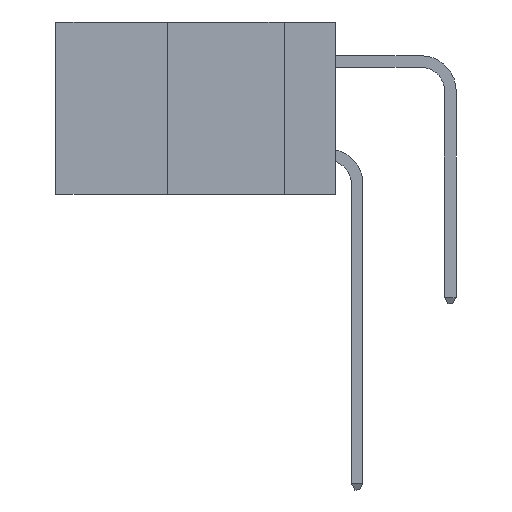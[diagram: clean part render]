
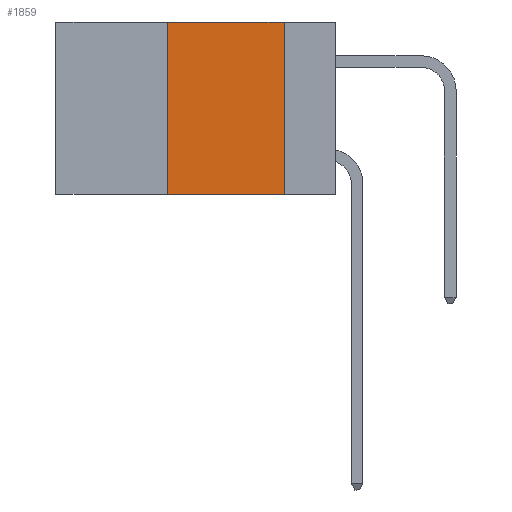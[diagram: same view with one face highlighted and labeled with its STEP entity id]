
A CAD part, left-side view. The second image highlights one B-rep face of the part: STEP entity #1859.
In plain terms, the highlighted planar face has unit normal (-1, 0, 0).
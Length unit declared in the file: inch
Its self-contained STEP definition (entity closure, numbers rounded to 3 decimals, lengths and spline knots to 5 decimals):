
#410 = VERTEX_POINT ( 'NONE', #22823 ) ;
#966 = EDGE_CURVE ( 'NONE', #22401, #4072, #22796, .T. ) ;
#1194 = CARTESIAN_POINT ( 'NONE',  ( 0., 0.11, 0. ) ) ;
#1469 = PLANE ( 'NONE',  #1845 ) ;
#1845 = AXIS2_PLACEMENT_3D ( 'NONE', #17821, #3337, #16053 ) ;
#1859 = ADVANCED_FACE ( 'NONE', ( #3425 ), #1469, .F. ) ;
#3337 = DIRECTION ( 'NONE',  ( 1., 0., 0. ) ) ;
#3425 = FACE_OUTER_BOUND ( 'NONE', #22972, .T. ) ;
#4072 = VERTEX_POINT ( 'NONE', #20283 ) ;
#4544 = CARTESIAN_POINT ( 'NONE',  ( 0., 0.11, 0. ) ) ;
#4611 = LINE ( 'NONE', #4544, #5171 ) ;
#5171 = VECTOR ( 'NONE', #17286, 39.37008 ) ;
#5440 = DIRECTION ( 'NONE',  ( 0., -1., 0. ) ) ;
#9307 = CARTESIAN_POINT ( 'NONE',  ( 0., 0.36, -0.37 ) ) ;
#10501 = ORIENTED_EDGE ( 'NONE', *, *, #19304, .F. ) ;
#11404 = CARTESIAN_POINT ( 'NONE',  ( 0., 0.36, 0. ) ) ;
#11487 = DIRECTION ( 'NONE',  ( 0., -1., 0. ) ) ;
#11617 = ORIENTED_EDGE ( 'NONE', *, *, #966, .F. ) ;
#11668 = LINE ( 'NONE', #14525, #16511 ) ;
#11678 = ORIENTED_EDGE ( 'NONE', *, *, #16087, .T. ) ;
#12528 = VECTOR ( 'NONE', #11487, 39.37008 ) ;
#13250 = DIRECTION ( 'NONE',  ( 0., 0., 1. ) ) ;
#14525 = CARTESIAN_POINT ( 'NONE',  ( 0., 0.6, 0. ) ) ;
#15628 = VERTEX_POINT ( 'NONE', #1194 ) ;
#15882 = EDGE_CURVE ( 'NONE', #4072, #15628, #11668, .T. ) ;
#16053 = DIRECTION ( 'NONE',  ( 0., 0., -1. ) ) ;
#16087 = EDGE_CURVE ( 'NONE', #22401, #410, #21070, .T. ) ;
#16117 = ORIENTED_EDGE ( 'NONE', *, *, #15882, .F. ) ;
#16511 = VECTOR ( 'NONE', #5440, 39.37008 ) ;
#16898 = CARTESIAN_POINT ( 'NONE',  ( 0., 0.6, -0.37 ) ) ;
#17286 = DIRECTION ( 'NONE',  ( 0., 0., -1. ) ) ;
#17821 = CARTESIAN_POINT ( 'NONE',  ( 0., 0.6, 0. ) ) ;
#17997 = VECTOR ( 'NONE', #13250, 39.37008 ) ;
#19304 = EDGE_CURVE ( 'NONE', #15628, #410, #4611, .T. ) ;
#20283 = CARTESIAN_POINT ( 'NONE',  ( 0., 0.36, 0. ) ) ;
#21070 = LINE ( 'NONE', #16898, #12528 ) ;
#22401 = VERTEX_POINT ( 'NONE', #9307 ) ;
#22796 = LINE ( 'NONE', #11404, #17997 ) ;
#22823 = CARTESIAN_POINT ( 'NONE',  ( 0., 0.11, -0.37 ) ) ;
#22972 = EDGE_LOOP ( 'NONE', ( #10501, #16117, #11617, #11678 ) ) ;
